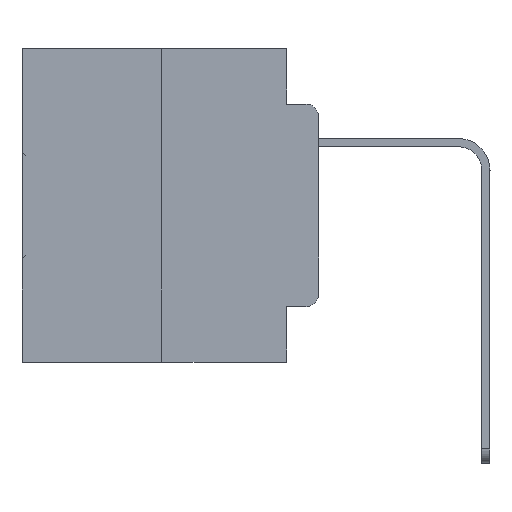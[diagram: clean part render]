
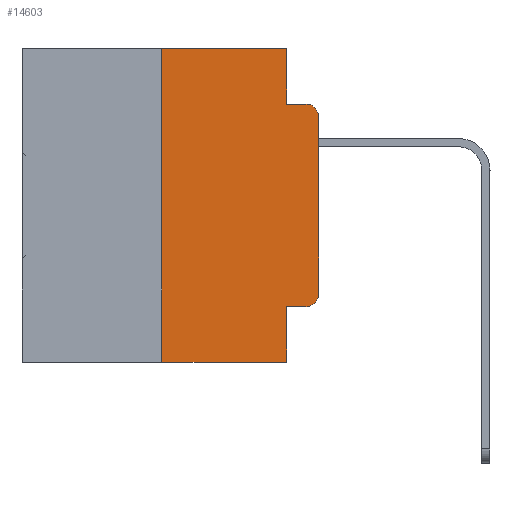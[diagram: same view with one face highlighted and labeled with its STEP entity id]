
A CAD part, left-side view. The second image highlights one B-rep face of the part: STEP entity #14603.
In plain terms, the highlighted planar face has unit normal (-1, 0, 0).
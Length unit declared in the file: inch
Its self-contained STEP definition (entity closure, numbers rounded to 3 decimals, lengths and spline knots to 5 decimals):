
#67 = CIRCLE ( 'NONE', #2168, 0.02 ) ;
#861 = EDGE_CURVE ( 'NONE', #31778, #21952, #11269, .T. ) ;
#1493 = EDGE_CURVE ( 'NONE', #15179, #31778, #25535, .T. ) ;
#2168 = AXIS2_PLACEMENT_3D ( 'NONE', #14703, #24954, #29871 ) ;
#2302 = CARTESIAN_POINT ( 'NONE',  ( 0., 0.02, -0.0885 ) ) ;
#2365 = DIRECTION ( 'NONE',  ( 0., -1., 0. ) ) ;
#2522 = EDGE_CURVE ( 'NONE', #31539, #3147, #25846, .T. ) ;
#3147 = VERTEX_POINT ( 'NONE', #8743 ) ;
#3987 = CARTESIAN_POINT ( 'NONE',  ( 0., 0., -0.1085 ) ) ;
#4186 = CARTESIAN_POINT ( 'NONE',  ( 0., 0.473, 0. ) ) ;
#4437 = DIRECTION ( 'NONE',  ( 0., -1., 0. ) ) ;
#4466 = CARTESIAN_POINT ( 'NONE',  ( 0., 0.051, 0. ) ) ;
#5323 = VERTEX_POINT ( 'NONE', #17144 ) ;
#5407 = VECTOR ( 'NONE', #2365, 39.37008 ) ;
#5835 = CARTESIAN_POINT ( 'NONE',  ( 0., 0.051, -0.0885 ) ) ;
#6010 = EDGE_CURVE ( 'NONE', #6403, #21952, #31839, .T. ) ;
#6403 = VERTEX_POINT ( 'NONE', #3987 ) ;
#6502 = EDGE_LOOP ( 'NONE', ( #12661, #16927, #19973, #13652, #30641, #27816, #11675, #9363, #25211, #12834 ) ) ;
#6711 = EDGE_CURVE ( 'NONE', #15636, #26467, #67, .T. ) ;
#6961 = DIRECTION ( 'NONE',  ( 1., 0., 0. ) ) ;
#7103 = EDGE_CURVE ( 'NONE', #31539, #5323, #16710, .T. ) ;
#8405 = DIRECTION ( 'NONE',  ( 0., 0., -1. ) ) ;
#8743 = CARTESIAN_POINT ( 'NONE',  ( 0., 0.25, 0. ) ) ;
#8913 = VECTOR ( 'NONE', #14049, 39.37008 ) ;
#9316 = DIRECTION ( 'NONE',  ( -1., 0., 0. ) ) ;
#9363 = ORIENTED_EDGE ( 'NONE', *, *, #25751, .F. ) ;
#9522 = EDGE_CURVE ( 'NONE', #3147, #15179, #12031, .T. ) ;
#10448 = VECTOR ( 'NONE', #29288, 39.37008 ) ;
#11269 = LINE ( 'NONE', #14483, #5407 ) ;
#11675 = ORIENTED_EDGE ( 'NONE', *, *, #7103, .T. ) ;
#11833 = DIRECTION ( 'NONE',  ( 0., 0., -1. ) ) ;
#11966 = DIRECTION ( 'NONE',  ( 0., 0., 1. ) ) ;
#12031 = LINE ( 'NONE', #4186, #8913 ) ;
#12173 = CARTESIAN_POINT ( 'NONE',  ( 0., 0.25, 0. ) ) ;
#12661 = ORIENTED_EDGE ( 'NONE', *, *, #15416, .T. ) ;
#12834 = ORIENTED_EDGE ( 'NONE', *, *, #6711, .T. ) ;
#13565 = CARTESIAN_POINT ( 'NONE',  ( 0., 0.473, -0.5 ) ) ;
#13652 = ORIENTED_EDGE ( 'NONE', *, *, #1493, .F. ) ;
#14049 = DIRECTION ( 'NONE',  ( 0., -1., 0. ) ) ;
#14141 = LINE ( 'NONE', #24050, #30039 ) ;
#14483 = CARTESIAN_POINT ( 'NONE',  ( 0., 0.051, -0.0885 ) ) ;
#14603 = ADVANCED_FACE ( 'NONE', ( #24901 ), #17325, .F. ) ;
#14643 = CARTESIAN_POINT ( 'NONE',  ( 0., 0.051, 0. ) ) ;
#14703 = CARTESIAN_POINT ( 'NONE',  ( 0., 0.02, -0.3915 ) ) ;
#15179 = VERTEX_POINT ( 'NONE', #14643 ) ;
#15416 = EDGE_CURVE ( 'NONE', #26467, #6403, #31894, .T. ) ;
#15636 = VERTEX_POINT ( 'NONE', #21607 ) ;
#16710 = LINE ( 'NONE', #13565, #20994 ) ;
#16927 = ORIENTED_EDGE ( 'NONE', *, *, #6010, .T. ) ;
#17144 = CARTESIAN_POINT ( 'NONE',  ( 0., 0.051, -0.5 ) ) ;
#17294 = VECTOR ( 'NONE', #11966, 39.37008 ) ;
#17325 = PLANE ( 'NONE',  #20317 ) ;
#18620 = VERTEX_POINT ( 'NONE', #30619 ) ;
#18639 = VECTOR ( 'NONE', #20546, 39.37008 ) ;
#19478 = LINE ( 'NONE', #23447, #31951 ) ;
#19555 = EDGE_CURVE ( 'NONE', #18620, #15636, #14141, .T. ) ;
#19973 = ORIENTED_EDGE ( 'NONE', *, *, #861, .F. ) ;
#20317 = AXIS2_PLACEMENT_3D ( 'NONE', #21791, #6961, #24310 ) ;
#20546 = DIRECTION ( 'NONE',  ( 0., 0., 1. ) ) ;
#20994 = VECTOR ( 'NONE', #31023, 39.37008 ) ;
#21607 = CARTESIAN_POINT ( 'NONE',  ( 0., 0.02, -0.4115 ) ) ;
#21791 = CARTESIAN_POINT ( 'NONE',  ( 0., 0.473, 0. ) ) ;
#21952 = VERTEX_POINT ( 'NONE', #2302 ) ;
#23447 = CARTESIAN_POINT ( 'NONE',  ( 0., 0.051, 0. ) ) ;
#24050 = CARTESIAN_POINT ( 'NONE',  ( 0., 0.051, -0.4115 ) ) ;
#24163 = CARTESIAN_POINT ( 'NONE',  ( 0., 0.02, -0.1085 ) ) ;
#24310 = DIRECTION ( 'NONE',  ( 0., 0., -1. ) ) ;
#24901 = FACE_OUTER_BOUND ( 'NONE', #6502, .T. ) ;
#24954 = DIRECTION ( 'NONE',  ( -1., 0., 0. ) ) ;
#25211 = ORIENTED_EDGE ( 'NONE', *, *, #19555, .T. ) ;
#25535 = LINE ( 'NONE', #4466, #10448 ) ;
#25751 = EDGE_CURVE ( 'NONE', #18620, #5323, #19478, .T. ) ;
#25846 = LINE ( 'NONE', #12173, #17294 ) ;
#26467 = VERTEX_POINT ( 'NONE', #27364 ) ;
#27364 = CARTESIAN_POINT ( 'NONE',  ( 0., 0., -0.3915 ) ) ;
#27816 = ORIENTED_EDGE ( 'NONE', *, *, #2522, .F. ) ;
#27855 = AXIS2_PLACEMENT_3D ( 'NONE', #24163, #9316, #11833 ) ;
#28476 = CARTESIAN_POINT ( 'NONE',  ( 0., 0., 0. ) ) ;
#29285 = CARTESIAN_POINT ( 'NONE',  ( 0., 0.25, -0.5 ) ) ;
#29288 = DIRECTION ( 'NONE',  ( 0., 0., -1. ) ) ;
#29871 = DIRECTION ( 'NONE',  ( 0., 0., -1. ) ) ;
#30039 = VECTOR ( 'NONE', #4437, 39.37008 ) ;
#30619 = CARTESIAN_POINT ( 'NONE',  ( 0., 0.051, -0.4115 ) ) ;
#30641 = ORIENTED_EDGE ( 'NONE', *, *, #9522, .F. ) ;
#31023 = DIRECTION ( 'NONE',  ( 0., -1., 0. ) ) ;
#31539 = VERTEX_POINT ( 'NONE', #29285 ) ;
#31778 = VERTEX_POINT ( 'NONE', #5835 ) ;
#31839 = CIRCLE ( 'NONE', #27855, 0.02 ) ;
#31894 = LINE ( 'NONE', #28476, #18639 ) ;
#31951 = VECTOR ( 'NONE', #8405, 39.37008 ) ;
